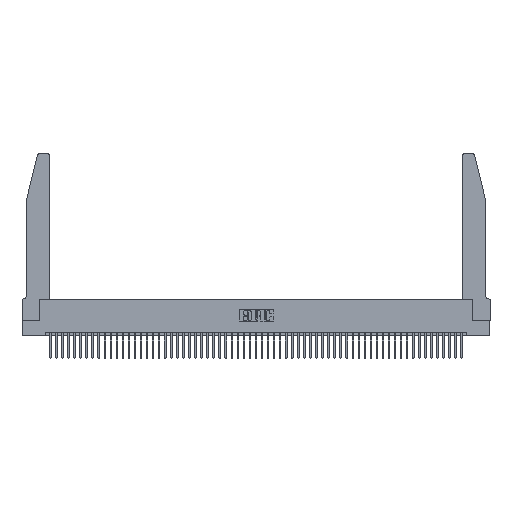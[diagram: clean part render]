
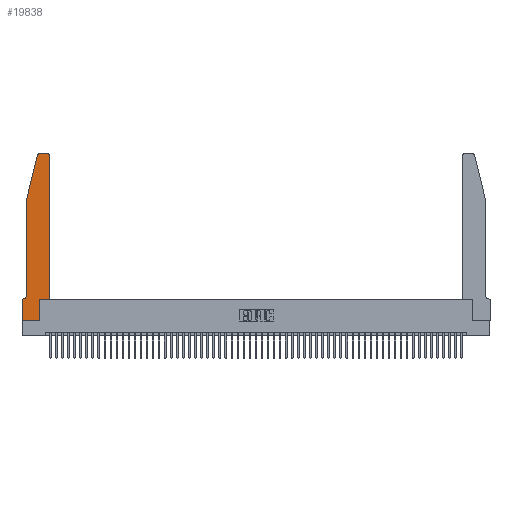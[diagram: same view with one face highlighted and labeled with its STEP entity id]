
A CAD part, top view. The second image highlights one B-rep face of the part: STEP entity #19838.
In plain terms, the highlighted planar face has unit normal (0, 0, 1).
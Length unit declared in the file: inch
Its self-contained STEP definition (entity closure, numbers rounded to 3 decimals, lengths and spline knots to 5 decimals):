
#24 = DIRECTION ( 'NONE',  ( 1., 0., 0. ) ) ;
#772 = AXIS2_PLACEMENT_3D ( 'NONE', #50882, #25357, #55144 ) ;
#989 = VECTOR ( 'NONE', #43661, 39.37008 ) ;
#1283 = VERTEX_POINT ( 'NONE', #37420 ) ;
#1976 = DIRECTION ( 'NONE',  ( 0., 0., 1. ) ) ;
#2766 = CARTESIAN_POINT ( 'NONE',  ( 0., 0., 0.37 ) ) ;
#4881 = VERTEX_POINT ( 'NONE', #9993 ) ;
#5129 = CARTESIAN_POINT ( 'NONE',  ( 0.0755, 0.35, 0.37 ) ) ;
#5682 = DIRECTION ( 'NONE',  ( -0.239, -0.971, 0. ) ) ;
#6012 = VECTOR ( 'NONE', #33644, 39.37008 ) ;
#6151 = EDGE_CURVE ( 'NONE', #45121, #33756, #41494, .T. ) ;
#6670 = LINE ( 'NONE', #34907, #39435 ) ;
#6897 = VECTOR ( 'NONE', #19619, 39.37008 ) ;
#8297 = VERTEX_POINT ( 'NONE', #32816 ) ;
#9192 = EDGE_CURVE ( 'NONE', #32436, #1283, #12422, .T. ) ;
#9710 = CARTESIAN_POINT ( 'NONE',  ( 0.2865, 0.35, 0.37 ) ) ;
#9716 = LINE ( 'NONE', #2766, #53726 ) ;
#9722 = DIRECTION ( 'NONE',  ( -1., 0., 0. ) ) ;
#9993 = CARTESIAN_POINT ( 'NONE',  ( 0.4505, 0.35, 0.37 ) ) ;
#10491 = ORIENTED_EDGE ( 'NONE', *, *, #24657, .T. ) ;
#12365 = LINE ( 'NONE', #14021, #32427 ) ;
#12422 = LINE ( 'NONE', #9710, #989 ) ;
#13262 = ORIENTED_EDGE ( 'NONE', *, *, #44396, .T. ) ;
#13844 = EDGE_CURVE ( 'NONE', #21294, #45005, #49841, .T. ) ;
#14021 = CARTESIAN_POINT ( 'NONE',  ( 0.2605, 2.75, 0.37 ) ) ;
#14477 = ORIENTED_EDGE ( 'NONE', *, *, #28951, .T. ) ;
#15434 = ORIENTED_EDGE ( 'NONE', *, *, #27865, .T. ) ;
#15801 = VECTOR ( 'NONE', #18033, 39.37008 ) ;
#16160 = ORIENTED_EDGE ( 'NONE', *, *, #30485, .T. ) ;
#16637 = CARTESIAN_POINT ( 'NONE',  ( 0.4505, 0.35, 0.37 ) ) ;
#17539 = VERTEX_POINT ( 'NONE', #33919 ) ;
#17805 = VECTOR ( 'NONE', #5682, 39.37008 ) ;
#18033 = DIRECTION ( 'NONE',  ( -1., 0., 0. ) ) ;
#19619 = DIRECTION ( 'NONE',  ( 0., -1., 0. ) ) ;
#19824 = VERTEX_POINT ( 'NONE', #46725 ) ;
#19838 = ADVANCED_FACE ( 'NONE', ( #42232 ), #55284, .T. ) ;
#19974 = DIRECTION ( 'NONE',  ( 0., -1., 0. ) ) ;
#20008 = ORIENTED_EDGE ( 'NONE', *, *, #13844, .T. ) ;
#20720 = CARTESIAN_POINT ( 'NONE',  ( 0.0055, 0.42, 0.37 ) ) ;
#20985 = ORIENTED_EDGE ( 'NONE', *, *, #54504, .T. ) ;
#21294 = VERTEX_POINT ( 'NONE', #43061 ) ;
#23832 = ORIENTED_EDGE ( 'NONE', *, *, #9192, .T. ) ;
#24217 = CARTESIAN_POINT ( 'NONE',  ( 0.2865, 0., 0.37 ) ) ;
#24657 = EDGE_CURVE ( 'NONE', #32755, #21294, #44144, .T. ) ;
#25025 = DIRECTION ( 'NONE',  ( -1., 0., 0. ) ) ;
#25357 = DIRECTION ( 'NONE',  ( 0., 0., 1. ) ) ;
#25505 = CARTESIAN_POINT ( 'NONE',  ( 0., 0.35, 0.37 ) ) ;
#25676 = DIRECTION ( 'NONE',  ( 0., 0., 1. ) ) ;
#26402 = ORIENTED_EDGE ( 'NONE', *, *, #46429, .T. ) ;
#26438 = CARTESIAN_POINT ( 'NONE',  ( 0.0755, 0.42, 0.37 ) ) ;
#26609 = CARTESIAN_POINT ( 'NONE',  ( 0.4505, 2.72, 0.37 ) ) ;
#27007 = CARTESIAN_POINT ( 'NONE',  ( 0.0755, 2., 0.37 ) ) ;
#27637 = CARTESIAN_POINT ( 'NONE',  ( 0.4205, 2.72, 0.37 ) ) ;
#27865 = EDGE_CURVE ( 'NONE', #17539, #8297, #51831, .T. ) ;
#28791 = LINE ( 'NONE', #16637, #6012 ) ;
#28951 = EDGE_CURVE ( 'NONE', #33756, #19824, #12365, .T. ) ;
#29188 = AXIS2_PLACEMENT_3D ( 'NONE', #20720, #50532, #25025 ) ;
#30207 = CARTESIAN_POINT ( 'NONE',  ( 0., 0.35, 0.37 ) ) ;
#30485 = EDGE_CURVE ( 'NONE', #8297, #32755, #52294, .T. ) ;
#30751 = ORIENTED_EDGE ( 'NONE', *, *, #41502, .T. ) ;
#31165 = CIRCLE ( 'NONE', #772, 0.03 ) ;
#31626 = ORIENTED_EDGE ( 'NONE', *, *, #6151, .T. ) ;
#31938 = DIRECTION ( 'NONE',  ( 1., 0., 0. ) ) ;
#32427 = VECTOR ( 'NONE', #9722, 39.37008 ) ;
#32436 = VERTEX_POINT ( 'NONE', #24217 ) ;
#32755 = VERTEX_POINT ( 'NONE', #26438 ) ;
#32816 = CARTESIAN_POINT ( 'NONE',  ( 0.0755, 2., 0.37 ) ) ;
#33644 = DIRECTION ( 'NONE',  ( 1., 0., 0. ) ) ;
#33756 = VERTEX_POINT ( 'NONE', #37360 ) ;
#33919 = CARTESIAN_POINT ( 'NONE',  ( 0.25487, 2.72718, 0.37 ) ) ;
#34907 = CARTESIAN_POINT ( 'NONE',  ( 0.4505, 0.35, 0.37 ) ) ;
#36666 = CARTESIAN_POINT ( 'NONE',  ( 0.0755, 2., 0.37 ) ) ;
#36756 = VERTEX_POINT ( 'NONE', #43376 ) ;
#36964 = EDGE_LOOP ( 'NONE', ( #14477, #20985, #15434, #16160, #10491, #20008, #30751, #26402, #23832, #47678, #13262, #31626 ) ) ;
#37360 = CARTESIAN_POINT ( 'NONE',  ( 0.4205, 2.75, 0.37 ) ) ;
#37420 = CARTESIAN_POINT ( 'NONE',  ( 0.2865, 0.35, 0.37 ) ) ;
#37938 = AXIS2_PLACEMENT_3D ( 'NONE', #27637, #1976, #31938 ) ;
#39194 = DIRECTION ( 'NONE',  ( 0., 1., 0. ) ) ;
#39435 = VECTOR ( 'NONE', #39194, 39.37008 ) ;
#39864 = LINE ( 'NONE', #45092, #49811 ) ;
#41194 = AXIS2_PLACEMENT_3D ( 'NONE', #25505, #25676, #24 ) ;
#41494 = CIRCLE ( 'NONE', #37938, 0.03 ) ;
#41502 = EDGE_CURVE ( 'NONE', #45005, #36756, #9716, .T. ) ;
#42232 = FACE_OUTER_BOUND ( 'NONE', #36964, .T. ) ;
#43061 = CARTESIAN_POINT ( 'NONE',  ( 0.0055, 0.35, 0.37 ) ) ;
#43376 = CARTESIAN_POINT ( 'NONE',  ( 0., 0., 0.37 ) ) ;
#43494 = EDGE_CURVE ( 'NONE', #1283, #4881, #28791, .T. ) ;
#43661 = DIRECTION ( 'NONE',  ( 0., 1., 0. ) ) ;
#44144 = CIRCLE ( 'NONE', #29188, 0.07 ) ;
#44396 = EDGE_CURVE ( 'NONE', #4881, #45121, #6670, .T. ) ;
#45005 = VERTEX_POINT ( 'NONE', #30207 ) ;
#45092 = CARTESIAN_POINT ( 'NONE',  ( 0., 0., 0.37 ) ) ;
#45121 = VERTEX_POINT ( 'NONE', #26609 ) ;
#46429 = EDGE_CURVE ( 'NONE', #36756, #32436, #39864, .T. ) ;
#46725 = CARTESIAN_POINT ( 'NONE',  ( 0.284, 2.75, 0.37 ) ) ;
#47678 = ORIENTED_EDGE ( 'NONE', *, *, #43494, .T. ) ;
#49371 = DIRECTION ( 'NONE',  ( 1., 0., 0. ) ) ;
#49811 = VECTOR ( 'NONE', #49371, 39.37008 ) ;
#49841 = LINE ( 'NONE', #5129, #15801 ) ;
#50532 = DIRECTION ( 'NONE',  ( 0., 0., -1. ) ) ;
#50882 = CARTESIAN_POINT ( 'NONE',  ( 0.284, 2.72, 0.37 ) ) ;
#51831 = LINE ( 'NONE', #27007, #17805 ) ;
#52294 = LINE ( 'NONE', #36666, #6897 ) ;
#53726 = VECTOR ( 'NONE', #19974, 39.37008 ) ;
#54504 = EDGE_CURVE ( 'NONE', #19824, #17539, #31165, .T. ) ;
#55144 = DIRECTION ( 'NONE',  ( 1., 0., 0. ) ) ;
#55284 = PLANE ( 'NONE',  #41194 ) ;
